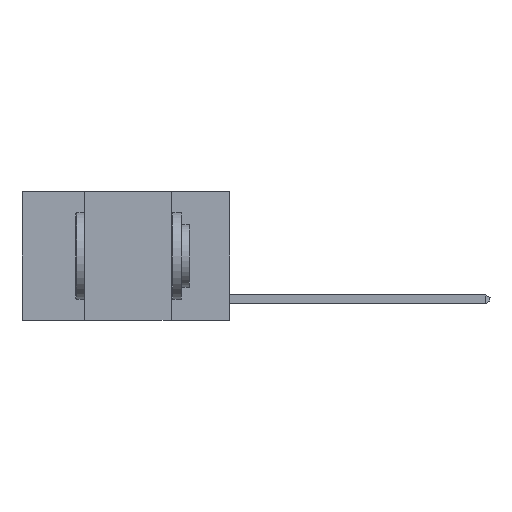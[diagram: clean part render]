
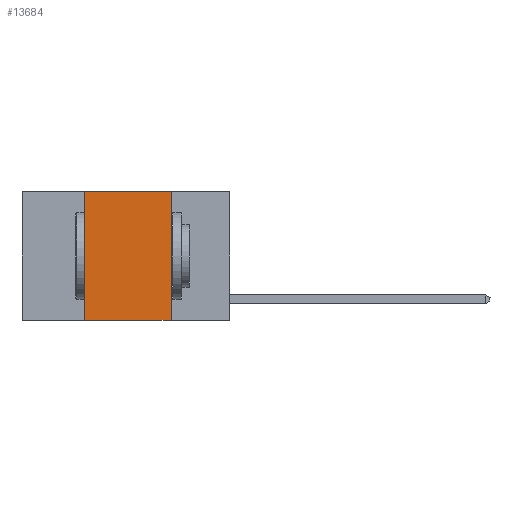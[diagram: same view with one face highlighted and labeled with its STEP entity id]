
A CAD part, left-side view. The second image highlights one B-rep face of the part: STEP entity #13684.
In plain terms, the highlighted planar face has unit normal (-1, 0, 0).
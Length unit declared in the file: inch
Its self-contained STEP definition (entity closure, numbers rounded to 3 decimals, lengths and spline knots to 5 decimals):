
#587 = LINE ( 'NONE', #7784, #29930 ) ;
#715 = PLANE ( 'NONE',  #3263 ) ;
#787 = VECTOR ( 'NONE', #6651, 39.37008 ) ;
#2668 = CARTESIAN_POINT ( 'NONE',  ( 0., 0.17, -0.37 ) ) ;
#3043 = DIRECTION ( 'NONE',  ( 0., 0., 1. ) ) ;
#3192 = CARTESIAN_POINT ( 'NONE',  ( 0., 0.42, 0. ) ) ;
#3263 = AXIS2_PLACEMENT_3D ( 'NONE', #5470, #10203, #26573 ) ;
#3399 = EDGE_CURVE ( 'NONE', #24591, #21668, #5184, .T. ) ;
#5184 = LINE ( 'NONE', #3192, #11711 ) ;
#5411 = CARTESIAN_POINT ( 'NONE',  ( 0., 0.17, 0. ) ) ;
#5470 = CARTESIAN_POINT ( 'NONE',  ( 0., 0.6, 0. ) ) ;
#5914 = EDGE_LOOP ( 'NONE', ( #21881, #6432, #23863, #16381 ) ) ;
#6432 = ORIENTED_EDGE ( 'NONE', *, *, #6442, .F. ) ;
#6442 = EDGE_CURVE ( 'NONE', #21668, #17540, #587, .T. ) ;
#6504 = CARTESIAN_POINT ( 'NONE',  ( 0., 0.6, -0.37 ) ) ;
#6651 = DIRECTION ( 'NONE',  ( 0., -1., 0. ) ) ;
#7042 = CARTESIAN_POINT ( 'NONE',  ( 0., 0.42, 0. ) ) ;
#7385 = CARTESIAN_POINT ( 'NONE',  ( 0., 0.17, 0. ) ) ;
#7784 = CARTESIAN_POINT ( 'NONE',  ( 0., 0.6, 0. ) ) ;
#8008 = DIRECTION ( 'NONE',  ( 0., 0., -1. ) ) ;
#10203 = DIRECTION ( 'NONE',  ( 1., 0., 0. ) ) ;
#11052 = VERTEX_POINT ( 'NONE', #2668 ) ;
#11711 = VECTOR ( 'NONE', #3043, 39.37008 ) ;
#12018 = CARTESIAN_POINT ( 'NONE',  ( 0., 0.42, -0.37 ) ) ;
#13034 = LINE ( 'NONE', #5411, #18913 ) ;
#13684 = ADVANCED_FACE ( 'NONE', ( #26719 ), #715, .F. ) ;
#16381 = ORIENTED_EDGE ( 'NONE', *, *, #24675, .T. ) ;
#17540 = VERTEX_POINT ( 'NONE', #7385 ) ;
#18913 = VECTOR ( 'NONE', #8008, 39.37008 ) ;
#21668 = VERTEX_POINT ( 'NONE', #7042 ) ;
#21881 = ORIENTED_EDGE ( 'NONE', *, *, #26245, .F. ) ;
#23863 = ORIENTED_EDGE ( 'NONE', *, *, #3399, .F. ) ;
#24591 = VERTEX_POINT ( 'NONE', #12018 ) ;
#24675 = EDGE_CURVE ( 'NONE', #24591, #11052, #25037, .T. ) ;
#25037 = LINE ( 'NONE', #6504, #787 ) ;
#26133 = DIRECTION ( 'NONE',  ( 0., -1., 0. ) ) ;
#26245 = EDGE_CURVE ( 'NONE', #17540, #11052, #13034, .T. ) ;
#26573 = DIRECTION ( 'NONE',  ( 0., 0., -1. ) ) ;
#26719 = FACE_OUTER_BOUND ( 'NONE', #5914, .T. ) ;
#29930 = VECTOR ( 'NONE', #26133, 39.37008 ) ;
